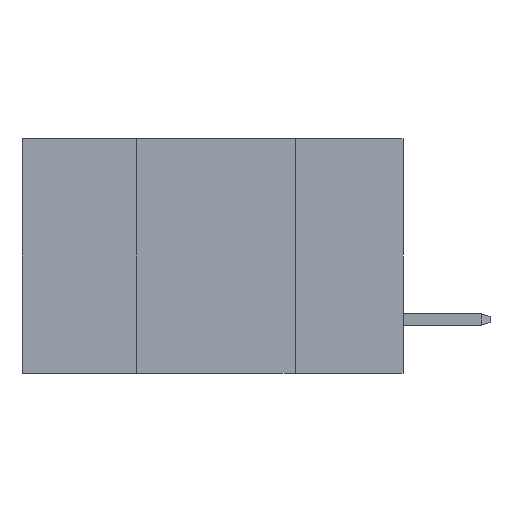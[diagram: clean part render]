
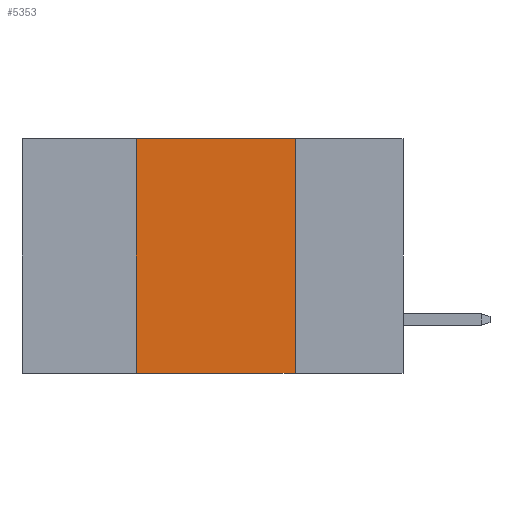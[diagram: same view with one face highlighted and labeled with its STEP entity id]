
A CAD part, left-side view. The second image highlights one B-rep face of the part: STEP entity #5353.
In plain terms, the highlighted planar face has unit normal (-1, 0, 0).
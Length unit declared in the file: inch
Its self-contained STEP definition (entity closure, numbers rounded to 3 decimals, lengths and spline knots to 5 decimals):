
#224 = CARTESIAN_POINT ( 'NONE',  ( 0., 0.6, -0.37 ) ) ;
#891 = LINE ( 'NONE', #224, #3101 ) ;
#1112 = VECTOR ( 'NONE', #2629, 39.37008 ) ;
#1409 = LINE ( 'NONE', #4618, #9170 ) ;
#1480 = DIRECTION ( 'NONE',  ( 0., -1., 0. ) ) ;
#1809 = DIRECTION ( 'NONE',  ( 0., -1., 0. ) ) ;
#2058 = CARTESIAN_POINT ( 'NONE',  ( 0., 0.42, 0. ) ) ;
#2133 = LINE ( 'NONE', #3739, #5460 ) ;
#2629 = DIRECTION ( 'NONE',  ( 0., 0., 1. ) ) ;
#2710 = VERTEX_POINT ( 'NONE', #6725 ) ;
#3101 = VECTOR ( 'NONE', #1809, 39.37008 ) ;
#3487 = CARTESIAN_POINT ( 'NONE',  ( 0., 0.42, 0. ) ) ;
#3739 = CARTESIAN_POINT ( 'NONE',  ( 0., 0.6, 0. ) ) ;
#4074 = ORIENTED_EDGE ( 'NONE', *, *, #8574, .F. ) ;
#4201 = CARTESIAN_POINT ( 'NONE',  ( 0., 0.42, -0.37 ) ) ;
#4341 = LINE ( 'NONE', #2058, #1112 ) ;
#4540 = CARTESIAN_POINT ( 'NONE',  ( 0., 0.6, 0. ) ) ;
#4562 = DIRECTION ( 'NONE',  ( 0., 0., -1. ) ) ;
#4618 = CARTESIAN_POINT ( 'NONE',  ( 0., 0.17, 0. ) ) ;
#4790 = ORIENTED_EDGE ( 'NONE', *, *, #7137, .F. ) ;
#5201 = CARTESIAN_POINT ( 'NONE',  ( 0., 0.17, 0. ) ) ;
#5215 = ORIENTED_EDGE ( 'NONE', *, *, #8498, .T. ) ;
#5246 = FACE_OUTER_BOUND ( 'NONE', #6995, .T. ) ;
#5315 = VERTEX_POINT ( 'NONE', #4201 ) ;
#5353 = ADVANCED_FACE ( 'NONE', ( #5246 ), #8187, .F. ) ;
#5429 = VERTEX_POINT ( 'NONE', #5201 ) ;
#5460 = VECTOR ( 'NONE', #1480, 39.37008 ) ;
#6353 = AXIS2_PLACEMENT_3D ( 'NONE', #4540, #6832, #8217 ) ;
#6725 = CARTESIAN_POINT ( 'NONE',  ( 0., 0.17, -0.37 ) ) ;
#6832 = DIRECTION ( 'NONE',  ( 1., 0., 0. ) ) ;
#6995 = EDGE_LOOP ( 'NONE', ( #4790, #7557, #4074, #5215 ) ) ;
#7137 = EDGE_CURVE ( 'NONE', #5429, #2710, #1409, .T. ) ;
#7557 = ORIENTED_EDGE ( 'NONE', *, *, #9677, .F. ) ;
#8187 = PLANE ( 'NONE',  #6353 ) ;
#8217 = DIRECTION ( 'NONE',  ( 0., 0., -1. ) ) ;
#8498 = EDGE_CURVE ( 'NONE', #5315, #2710, #891, .T. ) ;
#8574 = EDGE_CURVE ( 'NONE', #5315, #9009, #4341, .T. ) ;
#9009 = VERTEX_POINT ( 'NONE', #3487 ) ;
#9170 = VECTOR ( 'NONE', #4562, 39.37008 ) ;
#9677 = EDGE_CURVE ( 'NONE', #9009, #5429, #2133, .T. ) ;
